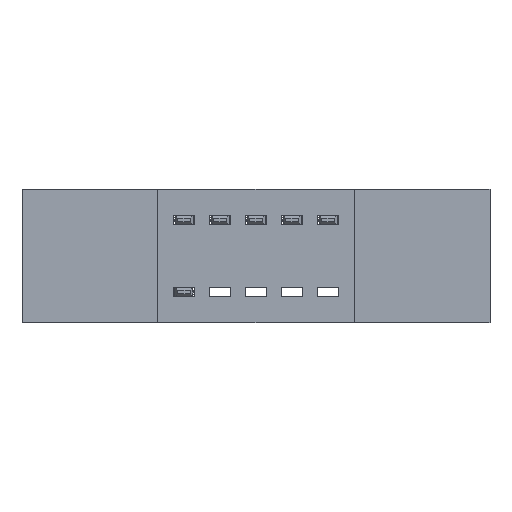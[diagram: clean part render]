
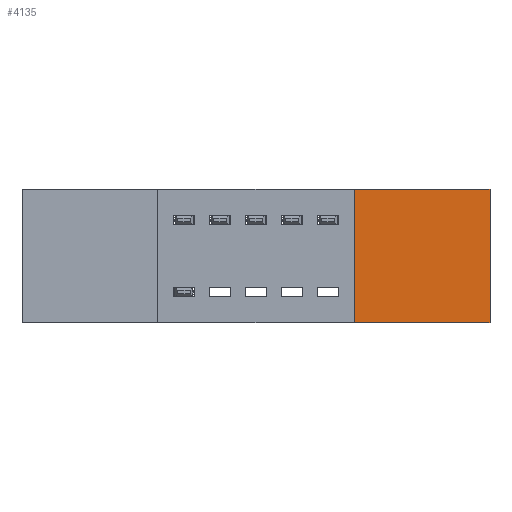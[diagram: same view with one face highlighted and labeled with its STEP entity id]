
A CAD part, front view. The second image highlights one B-rep face of the part: STEP entity #4135.
In plain terms, the highlighted planar face has unit normal (0, -1, 0).
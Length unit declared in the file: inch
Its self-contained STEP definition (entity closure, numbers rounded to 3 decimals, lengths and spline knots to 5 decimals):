
#653 = VERTEX_POINT ( 'NONE', #6002 ) ;
#1010 = ORIENTED_EDGE ( 'NONE', *, *, #3044, .F. ) ;
#1252 = EDGE_LOOP ( 'NONE', ( #1010, #4146, #3590, #2971 ) ) ;
#1602 = CARTESIAN_POINT ( 'NONE',  ( 0., 0., -0.37 ) ) ;
#1679 = VERTEX_POINT ( 'NONE', #5968 ) ;
#1759 = LINE ( 'NONE', #3635, #7505 ) ;
#1779 = VECTOR ( 'NONE', #5028, 39.37008 ) ;
#2072 = CARTESIAN_POINT ( 'NONE',  ( 0., 0., -0.37 ) ) ;
#2086 = VERTEX_POINT ( 'NONE', #3957 ) ;
#2155 = VECTOR ( 'NONE', #7436, 39.37008 ) ;
#2302 = EDGE_CURVE ( 'NONE', #653, #2086, #4578, .T. ) ;
#2361 = DIRECTION ( 'NONE',  ( 0., 0., -1. ) ) ;
#2971 = ORIENTED_EDGE ( 'NONE', *, *, #2302, .F. ) ;
#3044 = EDGE_CURVE ( 'NONE', #5409, #653, #1759, .T. ) ;
#3590 = ORIENTED_EDGE ( 'NONE', *, *, #7308, .F. ) ;
#3635 = CARTESIAN_POINT ( 'NONE',  ( 0.923, 0., -0.37 ) ) ;
#3918 = EDGE_CURVE ( 'NONE', #1679, #5409, #5919, .T. ) ;
#3936 = LINE ( 'NONE', #7424, #2155 ) ;
#3957 = CARTESIAN_POINT ( 'NONE',  ( 1.3, 0., 0. ) ) ;
#4135 = ADVANCED_FACE ( 'NONE', ( #7088 ), #7198, .T. ) ;
#4146 = ORIENTED_EDGE ( 'NONE', *, *, #3918, .F. ) ;
#4578 = LINE ( 'NONE', #5794, #1779 ) ;
#5028 = DIRECTION ( 'NONE',  ( 1., 0., 0. ) ) ;
#5155 = DIRECTION ( 'NONE',  ( 0., 0., 1. ) ) ;
#5409 = VERTEX_POINT ( 'NONE', #6408 ) ;
#5794 = CARTESIAN_POINT ( 'NONE',  ( 0., 0., 0. ) ) ;
#5919 = LINE ( 'NONE', #2072, #7014 ) ;
#5968 = CARTESIAN_POINT ( 'NONE',  ( 1.3, 0., -0.37 ) ) ;
#6002 = CARTESIAN_POINT ( 'NONE',  ( 0.923, 0., 0. ) ) ;
#6141 = AXIS2_PLACEMENT_3D ( 'NONE', #1602, #7395, #2361 ) ;
#6408 = CARTESIAN_POINT ( 'NONE',  ( 0.923, 0., -0.37 ) ) ;
#6735 = DIRECTION ( 'NONE',  ( -1., 0., 0. ) ) ;
#7014 = VECTOR ( 'NONE', #6735, 39.37008 ) ;
#7088 = FACE_OUTER_BOUND ( 'NONE', #1252, .T. ) ;
#7198 = PLANE ( 'NONE',  #6141 ) ;
#7308 = EDGE_CURVE ( 'NONE', #2086, #1679, #3936, .T. ) ;
#7395 = DIRECTION ( 'NONE',  ( 0., -1., 0. ) ) ;
#7424 = CARTESIAN_POINT ( 'NONE',  ( 1.3, 0., 0. ) ) ;
#7436 = DIRECTION ( 'NONE',  ( 0., 0., -1. ) ) ;
#7505 = VECTOR ( 'NONE', #5155, 39.37008 ) ;
